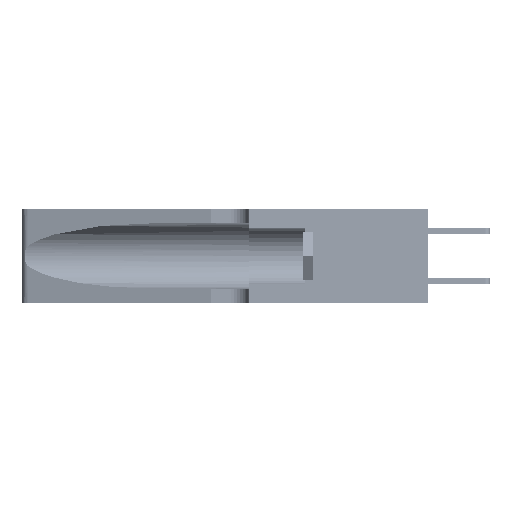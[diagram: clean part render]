
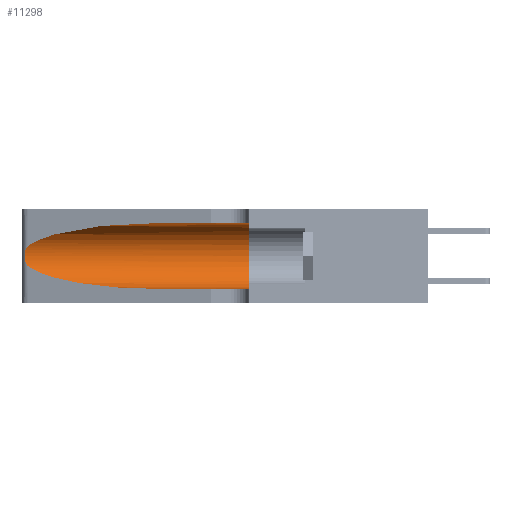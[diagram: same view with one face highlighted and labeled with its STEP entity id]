
A CAD part, left-side view. The second image highlights one B-rep face of the part: STEP entity #11298.
In plain terms, the highlighted cylindrical face has radius 3.308 mm (diameter 6.617 mm), a partial arc.
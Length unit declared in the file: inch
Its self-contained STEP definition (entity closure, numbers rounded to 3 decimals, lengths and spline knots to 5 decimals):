
#1581 = VECTOR ( 'NONE', #29279, 39.37008 ) ;
#1614 = CARTESIAN_POINT ( 'NONE',  ( 0.25487, 1.22718, 0.14631 ) ) ;
#2871 = CARTESIAN_POINT ( 'NONE',  ( 0.18966, 0.96281, 0.31525 ) ) ;
#2981 =( BOUNDED_CURVE ( )  B_SPLINE_CURVE ( 3, ( #27410, #27246, #27572, #4990 ),
 .UNSPECIFIED., .F., .F. ) 
 B_SPLINE_CURVE_WITH_KNOTS ( ( 4, 4 ),
 ( 3.44316, 4.71239 ),
 .UNSPECIFIED. ) 
 CURVE ( )  GEOMETRIC_REPRESENTATION_ITEM ( )  RATIONAL_B_SPLINE_CURVE ( ( 1., 0.87, 0.87, 1. ) ) 
 REPRESENTATION_ITEM ( '' )  );
#3527 = VERTEX_POINT ( 'NONE', #46555 ) ;
#4737 = VERTEX_POINT ( 'NONE', #29459 ) ;
#4990 = CARTESIAN_POINT ( 'NONE',  ( 0.1305, 0.72297, 0.05475 ) ) ;
#6140 = CIRCLE ( 'NONE', #36978, 0.13025 ) ;
#6209 = DIRECTION ( 'NONE',  ( 0., -1., 0. ) ) ;
#8878 = CARTESIAN_POINT ( 'NONE',  ( 0.25787, 1.23484, 0.2124 ) ) ;
#9201 = CARTESIAN_POINT ( 'NONE',  ( 0.26075, 1.23896, 0.178 ) ) ;
#9332 = VERTEX_POINT ( 'NONE', #40308 ) ;
#9517 = CARTESIAN_POINT ( 'NONE',  ( 0.25639, 1.23184, 0.21858 ) ) ;
#9949 = CARTESIAN_POINT ( 'NONE',  ( 0.1305, 0.35, 0.185 ) ) ;
#10260 = CARTESIAN_POINT ( 'NONE',  ( 0.1305, 0.72297, 0.31525 ) ) ;
#11298 = ADVANCED_FACE ( 'NONE', ( #19518 ), #45208, .F. ) ;
#11397 = LINE ( 'NONE', #28952, #1581 ) ;
#12330 = VECTOR ( 'NONE', #6209, 39.37008 ) ;
#12772 = CARTESIAN_POINT ( 'NONE',  ( 0.25639, 1.23186, 0.15144 ) ) ;
#12841 = DIRECTION ( 'NONE',  ( 0., 0., -1. ) ) ;
#14945 = AXIS2_PLACEMENT_3D ( 'NONE', #31846, #20758, #12841 ) ;
#16511 = CARTESIAN_POINT ( 'NONE',  ( 0.1305, 0.72297, 0.05475 ) ) ;
#17122 = CARTESIAN_POINT ( 'NONE',  ( 0.25487, 1.22718, 0.22369 ) ) ;
#18809 = ORIENTED_EDGE ( 'NONE', *, *, #46127, .T. ) ;
#19518 = FACE_OUTER_BOUND ( 'NONE', #26649, .T. ) ;
#19915 = CARTESIAN_POINT ( 'NONE',  ( 0.25555, 1.22993, 0.14849 ) ) ;
#20758 = DIRECTION ( 'NONE',  ( 0., -1., 0. ) ) ;
#22427 = EDGE_CURVE ( 'NONE', #25266, #9332, #11397, .T. ) ;
#23378 = EDGE_CURVE ( 'NONE', #4737, #34851, #2981, .T. ) ;
#23708 = CARTESIAN_POINT ( 'NONE',  ( 0.25856, 1.23593, 0.16098 ) ) ;
#24210 = CARTESIAN_POINT ( 'NONE',  ( 0.26018, 1.23835, 0.19895 ) ) ;
#24972 = VERTEX_POINT ( 'NONE', #30376 ) ;
#24974 = DIRECTION ( 'NONE',  ( 0., 0., 1. ) ) ;
#25266 = VERTEX_POINT ( 'NONE', #31980 ) ;
#25459 = ORIENTED_EDGE ( 'NONE', *, *, #22427, .F. ) ;
#26649 = EDGE_LOOP ( 'NONE', ( #46430, #18809, #40407, #29150, #35156, #25459 ) ) ;
#27246 = CARTESIAN_POINT ( 'NONE',  ( 0.2373, 1.15595, 0.08982 ) ) ;
#27410 = CARTESIAN_POINT ( 'NONE',  ( 0.25487, 1.22718, 0.14631 ) ) ;
#27572 = CARTESIAN_POINT ( 'NONE',  ( 0.18966, 0.96281, 0.05475 ) ) ;
#28952 = CARTESIAN_POINT ( 'NONE',  ( 0.1305, 1.61858, 0.31525 ) ) ;
#29150 = ORIENTED_EDGE ( 'NONE', *, *, #45069, .T. ) ;
#29279 = DIRECTION ( 'NONE',  ( 0., -1., 0. ) ) ;
#29459 = CARTESIAN_POINT ( 'NONE',  ( 0.25487, 1.22718, 0.14631 ) ) ;
#30376 = CARTESIAN_POINT ( 'NONE',  ( 0.25487, 1.22718, 0.22369 ) ) ;
#30637 = EDGE_CURVE ( 'NONE', #9332, #3527, #6140, .T. ) ;
#31830 = CARTESIAN_POINT ( 'NONE',  ( 0.25487, 1.22718, 0.22369 ) ) ;
#31846 = CARTESIAN_POINT ( 'NONE',  ( 0.1305, 1.61858, 0.185 ) ) ;
#31980 = CARTESIAN_POINT ( 'NONE',  ( 0.1305, 0.72297, 0.31525 ) ) ;
#34481 = LINE ( 'NONE', #39104, #12330 ) ;
#34851 = VERTEX_POINT ( 'NONE', #16511 ) ;
#35156 = ORIENTED_EDGE ( 'NONE', *, *, #30637, .F. ) ;
#35574 = CARTESIAN_POINT ( 'NONE',  ( 0.26075, 1.23896, 0.19203 ) ) ;
#36002 = DIRECTION ( 'NONE',  ( 0., 1., 0. ) ) ;
#36978 = AXIS2_PLACEMENT_3D ( 'NONE', #9949, #36002, #24974 ) ;
#39104 = CARTESIAN_POINT ( 'NONE',  ( 0.1305, 1.61858, 0.05475 ) ) ;
#39450 = CARTESIAN_POINT ( 'NONE',  ( 0.2373, 1.15595, 0.28018 ) ) ;
#40308 = CARTESIAN_POINT ( 'NONE',  ( 0.1305, 0.35, 0.31525 ) ) ;
#40407 = ORIENTED_EDGE ( 'NONE', *, *, #23378, .T. ) ;
#42608 = CARTESIAN_POINT ( 'NONE',  ( 0.25555, 1.22994, 0.2215 ) ) ;
#42635 =( BOUNDED_CURVE ( )  B_SPLINE_CURVE ( 3, ( #10260, #2871, #39450, #17122 ),
 .UNSPECIFIED., .F., .T. ) 
 B_SPLINE_CURVE_WITH_KNOTS ( ( 4, 4 ),
 ( 1.5708, 2.84003 ),
 .UNSPECIFIED. ) 
 CURVE ( )  GEOMETRIC_REPRESENTATION_ITEM ( )  RATIONAL_B_SPLINE_CURVE ( ( 1., 0.87, 0.87, 1. ) ) 
 REPRESENTATION_ITEM ( '' )  );
#42777 = CARTESIAN_POINT ( 'NONE',  ( 0.26017, 1.23833, 0.17102 ) ) ;
#45069 = EDGE_CURVE ( 'NONE', #34851, #3527, #34481, .T. ) ;
#45208 = CYLINDRICAL_SURFACE ( 'NONE', #14945, 0.13025 ) ;
#46019 = CARTESIAN_POINT ( 'NONE',  ( 0.25854, 1.2359, 0.20912 ) ) ;
#46127 = EDGE_CURVE ( 'NONE', #24972, #4737, #47697, .T. ) ;
#46351 = CARTESIAN_POINT ( 'NONE',  ( 0.25789, 1.23486, 0.15765 ) ) ;
#46430 = ORIENTED_EDGE ( 'NONE', *, *, #47279, .T. ) ;
#46555 = CARTESIAN_POINT ( 'NONE',  ( 0.1305, 0.35, 0.05475 ) ) ;
#47279 = EDGE_CURVE ( 'NONE', #25266, #24972, #42635, .T. ) ;
#47697 = B_SPLINE_CURVE_WITH_KNOTS ( 'NONE', 3,
 ( #31830, #42608, #9517, #8878, #46019, #24210, #35574, #9201, #42777, #23708, #46351, #12772, #19915, #1614 ),
 .UNSPECIFIED., .F., .F.,
 ( 4, 2, 2, 2, 2, 2, 4 ),
 ( 0., 0.00027, 0.00053, 0.00107, 0.0016, 0.00187, 0.00214 ),
 .UNSPECIFIED. ) ;
